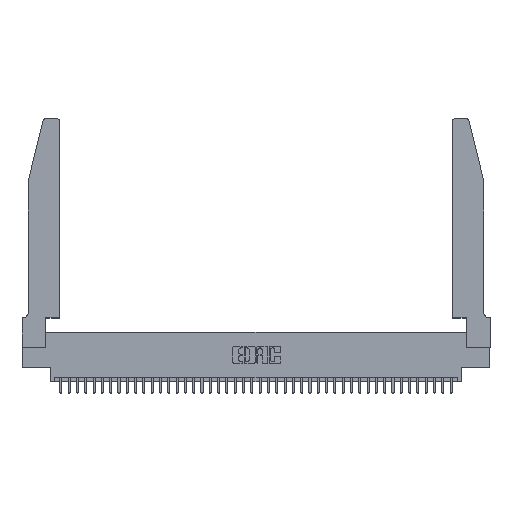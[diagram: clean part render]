
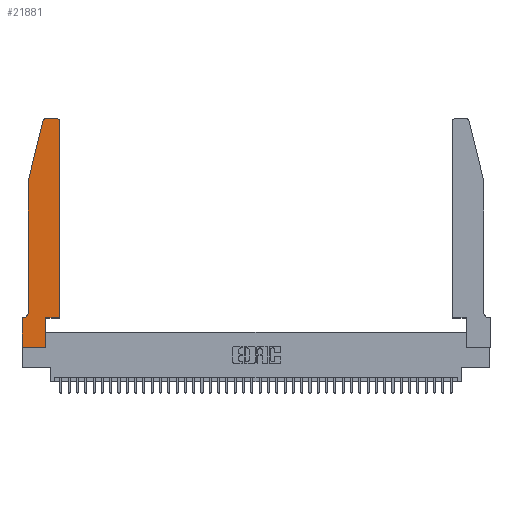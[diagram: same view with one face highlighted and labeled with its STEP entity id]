
A CAD part, top view. The second image highlights one B-rep face of the part: STEP entity #21881.
In plain terms, the highlighted planar face has unit normal (0, 0, 1).
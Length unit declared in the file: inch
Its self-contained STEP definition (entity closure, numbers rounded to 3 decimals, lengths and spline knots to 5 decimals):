
#18 = VERTEX_POINT ( 'NONE', #9783 ) ;
#1138 = VECTOR ( 'NONE', #36147, 39.37008 ) ;
#1248 = VECTOR ( 'NONE', #18758, 39.37008 ) ;
#1671 = CARTESIAN_POINT ( 'NONE',  ( 0.25487, 2.72718, 0.37 ) ) ;
#1939 = ORIENTED_EDGE ( 'NONE', *, *, #32655, .T. ) ;
#3372 = CARTESIAN_POINT ( 'NONE',  ( 0.0055, 0.35, 0.37 ) ) ;
#3914 = ORIENTED_EDGE ( 'NONE', *, *, #7506, .T. ) ;
#4011 = FACE_OUTER_BOUND ( 'NONE', #28541, .T. ) ;
#4072 = VERTEX_POINT ( 'NONE', #8709 ) ;
#4701 = DIRECTION ( 'NONE',  ( -1., 0., 0. ) ) ;
#5464 = CARTESIAN_POINT ( 'NONE',  ( 0.284, 2.72, 0.37 ) ) ;
#5634 = LINE ( 'NONE', #41284, #25286 ) ;
#5716 = LINE ( 'NONE', #34634, #38606 ) ;
#5997 = ORIENTED_EDGE ( 'NONE', *, *, #30454, .T. ) ;
#6452 = VERTEX_POINT ( 'NONE', #35059 ) ;
#6468 = DIRECTION ( 'NONE',  ( 1., 0., 0. ) ) ;
#7506 = EDGE_CURVE ( 'NONE', #4072, #18, #34528, .T. ) ;
#7990 = CARTESIAN_POINT ( 'NONE',  ( 0.0755, 0.42, 0.37 ) ) ;
#8051 = VECTOR ( 'NONE', #4701, 39.37008 ) ;
#8709 = CARTESIAN_POINT ( 'NONE',  ( 0.4505, 2.72, 0.37 ) ) ;
#8715 = ORIENTED_EDGE ( 'NONE', *, *, #33442, .T. ) ;
#8717 = DIRECTION ( 'NONE',  ( 0., 1., 0. ) ) ;
#8995 = ORIENTED_EDGE ( 'NONE', *, *, #37768, .T. ) ;
#9027 = CARTESIAN_POINT ( 'NONE',  ( 0., 0.35, 0.37 ) ) ;
#9202 = CARTESIAN_POINT ( 'NONE',  ( 0.4205, 2.72, 0.37 ) ) ;
#9783 = CARTESIAN_POINT ( 'NONE',  ( 0.4205, 2.75, 0.37 ) ) ;
#11802 = CARTESIAN_POINT ( 'NONE',  ( 0., 0.35, 0.37 ) ) ;
#13819 = ORIENTED_EDGE ( 'NONE', *, *, #28284, .T. ) ;
#14064 = VERTEX_POINT ( 'NONE', #32716 ) ;
#14736 = ORIENTED_EDGE ( 'NONE', *, *, #34469, .T. ) ;
#15628 = DIRECTION ( 'NONE',  ( 0., 0., 1. ) ) ;
#16674 = VERTEX_POINT ( 'NONE', #28333 ) ;
#16702 = VECTOR ( 'NONE', #29352, 39.37008 ) ;
#17356 = DIRECTION ( 'NONE',  ( -0.239, -0.971, 0. ) ) ;
#17645 = VECTOR ( 'NONE', #17356, 39.37008 ) ;
#18189 = VERTEX_POINT ( 'NONE', #26418 ) ;
#18739 = LINE ( 'NONE', #38474, #23788 ) ;
#18758 = DIRECTION ( 'NONE',  ( 0., -1., 0. ) ) ;
#18801 = VERTEX_POINT ( 'NONE', #26060 ) ;
#19050 = VERTEX_POINT ( 'NONE', #1671 ) ;
#19206 = LINE ( 'NONE', #39503, #16702 ) ;
#19218 = CARTESIAN_POINT ( 'NONE',  ( 0.4505, 0.35, 0.37 ) ) ;
#21434 = DIRECTION ( 'NONE',  ( -1., 0., 0. ) ) ;
#21571 = DIRECTION ( 'NONE',  ( 1., 0., 0. ) ) ;
#21881 = ADVANCED_FACE ( 'NONE', ( #4011 ), #31107, .T. ) ;
#22678 = LINE ( 'NONE', #29501, #17645 ) ;
#23179 = ORIENTED_EDGE ( 'NONE', *, *, #39988, .T. ) ;
#23788 = VECTOR ( 'NONE', #41696, 39.37008 ) ;
#24042 = CARTESIAN_POINT ( 'NONE',  ( 0.2605, 2.75, 0.37 ) ) ;
#25286 = VECTOR ( 'NONE', #38193, 39.37008 ) ;
#25299 = LINE ( 'NONE', #19218, #1138 ) ;
#25490 = EDGE_CURVE ( 'NONE', #36312, #32163, #36520, .T. ) ;
#25847 = DIRECTION ( 'NONE',  ( 0., -1., 0. ) ) ;
#26060 = CARTESIAN_POINT ( 'NONE',  ( 0.2865, 0., 0.37 ) ) ;
#26281 = CARTESIAN_POINT ( 'NONE',  ( 0., 0., 0.37 ) ) ;
#26383 = EDGE_CURVE ( 'NONE', #32163, #30755, #18739, .T. ) ;
#26418 = CARTESIAN_POINT ( 'NONE',  ( 0.4505, 0.35, 0.37 ) ) ;
#26499 = AXIS2_PLACEMENT_3D ( 'NONE', #40783, #27632, #21434 ) ;
#27436 = LINE ( 'NONE', #26281, #38566 ) ;
#27632 = DIRECTION ( 'NONE',  ( 0., 0., -1. ) ) ;
#27893 = ORIENTED_EDGE ( 'NONE', *, *, #25490, .T. ) ;
#28058 = AXIS2_PLACEMENT_3D ( 'NONE', #9202, #37689, #6468 ) ;
#28284 = EDGE_CURVE ( 'NONE', #14064, #18801, #5634, .T. ) ;
#28333 = CARTESIAN_POINT ( 'NONE',  ( 0.284, 2.75, 0.37 ) ) ;
#28541 = EDGE_LOOP ( 'NONE', ( #36103, #1939, #5997, #8995, #27893, #28994, #36351, #13819, #14736, #23179, #8715, #3914 ) ) ;
#28862 = AXIS2_PLACEMENT_3D ( 'NONE', #5464, #15628, #21571 ) ;
#28994 = ORIENTED_EDGE ( 'NONE', *, *, #26383, .T. ) ;
#29352 = DIRECTION ( 'NONE',  ( 0., 1., 0. ) ) ;
#29501 = CARTESIAN_POINT ( 'NONE',  ( 0.0755, 2., 0.37 ) ) ;
#30454 = EDGE_CURVE ( 'NONE', #19050, #37577, #22678, .T. ) ;
#30755 = VERTEX_POINT ( 'NONE', #9027 ) ;
#30777 = CARTESIAN_POINT ( 'NONE',  ( 0.0755, 2., 0.37 ) ) ;
#31107 = PLANE ( 'NONE',  #37842 ) ;
#31476 = CARTESIAN_POINT ( 'NONE',  ( 0.0755, 2., 0.37 ) ) ;
#32163 = VERTEX_POINT ( 'NONE', #3372 ) ;
#32655 = EDGE_CURVE ( 'NONE', #16674, #19050, #35625, .T. ) ;
#32716 = CARTESIAN_POINT ( 'NONE',  ( 0., 0., 0.37 ) ) ;
#33442 = EDGE_CURVE ( 'NONE', #18189, #4072, #5716, .T. ) ;
#33776 = EDGE_CURVE ( 'NONE', #30755, #14064, #27436, .T. ) ;
#34049 = LINE ( 'NONE', #31476, #1248 ) ;
#34469 = EDGE_CURVE ( 'NONE', #18801, #6452, #19206, .T. ) ;
#34528 = CIRCLE ( 'NONE', #28058, 0.03 ) ;
#34634 = CARTESIAN_POINT ( 'NONE',  ( 0.4505, 0.35, 0.37 ) ) ;
#35059 = CARTESIAN_POINT ( 'NONE',  ( 0.2865, 0.35, 0.37 ) ) ;
#35120 = EDGE_CURVE ( 'NONE', #18, #16674, #39335, .T. ) ;
#35625 = CIRCLE ( 'NONE', #28862, 0.03 ) ;
#36103 = ORIENTED_EDGE ( 'NONE', *, *, #35120, .T. ) ;
#36147 = DIRECTION ( 'NONE',  ( 1., 0., 0. ) ) ;
#36312 = VERTEX_POINT ( 'NONE', #7990 ) ;
#36351 = ORIENTED_EDGE ( 'NONE', *, *, #33776, .T. ) ;
#36520 = CIRCLE ( 'NONE', #26499, 0.07 ) ;
#37577 = VERTEX_POINT ( 'NONE', #30777 ) ;
#37689 = DIRECTION ( 'NONE',  ( 0., 0., 1. ) ) ;
#37744 = DIRECTION ( 'NONE',  ( 1., 0., 0. ) ) ;
#37768 = EDGE_CURVE ( 'NONE', #37577, #36312, #34049, .T. ) ;
#37842 = AXIS2_PLACEMENT_3D ( 'NONE', #11802, #40838, #37744 ) ;
#38193 = DIRECTION ( 'NONE',  ( 1., 0., 0. ) ) ;
#38474 = CARTESIAN_POINT ( 'NONE',  ( 0.0755, 0.35, 0.37 ) ) ;
#38566 = VECTOR ( 'NONE', #25847, 39.37008 ) ;
#38606 = VECTOR ( 'NONE', #8717, 39.37008 ) ;
#39335 = LINE ( 'NONE', #24042, #8051 ) ;
#39503 = CARTESIAN_POINT ( 'NONE',  ( 0.2865, 0.35, 0.37 ) ) ;
#39988 = EDGE_CURVE ( 'NONE', #6452, #18189, #25299, .T. ) ;
#40783 = CARTESIAN_POINT ( 'NONE',  ( 0.0055, 0.42, 0.37 ) ) ;
#40838 = DIRECTION ( 'NONE',  ( 0., 0., 1. ) ) ;
#41284 = CARTESIAN_POINT ( 'NONE',  ( 0., 0., 0.37 ) ) ;
#41696 = DIRECTION ( 'NONE',  ( -1., 0., 0. ) ) ;
